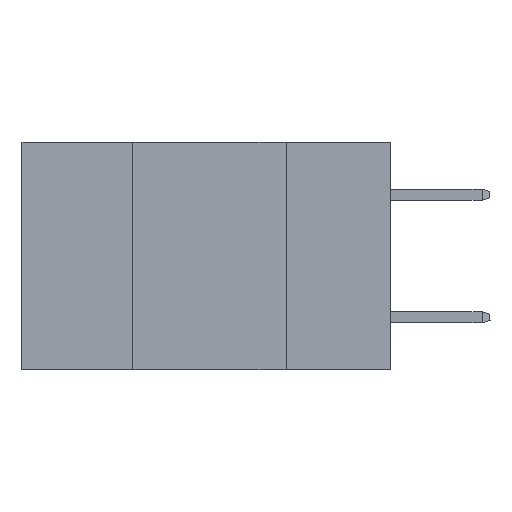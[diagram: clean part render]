
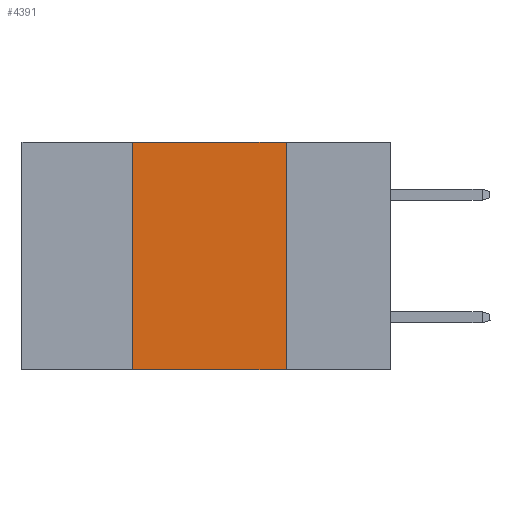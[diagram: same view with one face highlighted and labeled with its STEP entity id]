
A CAD part, left-side view. The second image highlights one B-rep face of the part: STEP entity #4391.
In plain terms, the highlighted planar face has unit normal (-1, 0, 0).
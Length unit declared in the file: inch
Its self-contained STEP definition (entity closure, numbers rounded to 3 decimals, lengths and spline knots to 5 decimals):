
#4319 = LINE ( 'NONE', #31485, #32512 ) ;
#4391 = ADVANCED_FACE ( 'NONE', ( #8613 ), #22609, .F. ) ;
#6191 = DIRECTION ( 'NONE',  ( 0., 0., -1. ) ) ;
#6222 = VERTEX_POINT ( 'NONE', #35526 ) ;
#8613 = FACE_OUTER_BOUND ( 'NONE', #30543, .T. ) ;
#12079 = VERTEX_POINT ( 'NONE', #28412 ) ;
#12082 = ORIENTED_EDGE ( 'NONE', *, *, #20210, .F. ) ;
#14172 = DIRECTION ( 'NONE',  ( 1., 0., 0. ) ) ;
#15584 = VERTEX_POINT ( 'NONE', #23538 ) ;
#16679 = CARTESIAN_POINT ( 'NONE',  ( 0., 0.6, -0.37 ) ) ;
#17180 = ORIENTED_EDGE ( 'NONE', *, *, #30322, .F. ) ;
#17472 = DIRECTION ( 'NONE',  ( 0., 0., 1. ) ) ;
#20210 = EDGE_CURVE ( 'NONE', #15584, #6222, #4319, .T. ) ;
#20642 = LINE ( 'NONE', #32106, #34933 ) ;
#22348 = CARTESIAN_POINT ( 'NONE',  ( 0., 0.17, -0.37 ) ) ;
#22609 = PLANE ( 'NONE',  #31688 ) ;
#23070 = CARTESIAN_POINT ( 'NONE',  ( 0., 0.6, 0. ) ) ;
#23356 = CARTESIAN_POINT ( 'NONE',  ( 0., 0.17, 0. ) ) ;
#23538 = CARTESIAN_POINT ( 'NONE',  ( 0., 0.42, -0.37 ) ) ;
#23602 = DIRECTION ( 'NONE',  ( 0., -1., 0. ) ) ;
#24228 = LINE ( 'NONE', #23356, #25144 ) ;
#25083 = DIRECTION ( 'NONE',  ( 0., -1., 0. ) ) ;
#25144 = VECTOR ( 'NONE', #6191, 39.37008 ) ;
#26761 = EDGE_CURVE ( 'NONE', #15584, #36620, #32567, .T. ) ;
#28075 = VECTOR ( 'NONE', #25083, 39.37008 ) ;
#28412 = CARTESIAN_POINT ( 'NONE',  ( 0., 0.17, 0. ) ) ;
#30322 = EDGE_CURVE ( 'NONE', #6222, #12079, #20642, .T. ) ;
#30333 = EDGE_CURVE ( 'NONE', #12079, #36620, #24228, .T. ) ;
#30543 = EDGE_LOOP ( 'NONE', ( #31820, #17180, #12082, #33447 ) ) ;
#31448 = DIRECTION ( 'NONE',  ( 0., 0., -1. ) ) ;
#31485 = CARTESIAN_POINT ( 'NONE',  ( 0., 0.42, 0. ) ) ;
#31688 = AXIS2_PLACEMENT_3D ( 'NONE', #23070, #14172, #31448 ) ;
#31820 = ORIENTED_EDGE ( 'NONE', *, *, #30333, .F. ) ;
#32106 = CARTESIAN_POINT ( 'NONE',  ( 0., 0.6, 0. ) ) ;
#32512 = VECTOR ( 'NONE', #17472, 39.37008 ) ;
#32567 = LINE ( 'NONE', #16679, #28075 ) ;
#33447 = ORIENTED_EDGE ( 'NONE', *, *, #26761, .T. ) ;
#34933 = VECTOR ( 'NONE', #23602, 39.37008 ) ;
#35526 = CARTESIAN_POINT ( 'NONE',  ( 0., 0.42, 0. ) ) ;
#36620 = VERTEX_POINT ( 'NONE', #22348 ) ;
